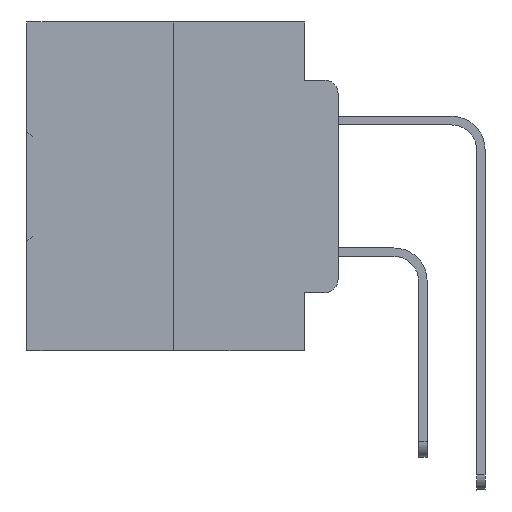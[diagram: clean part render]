
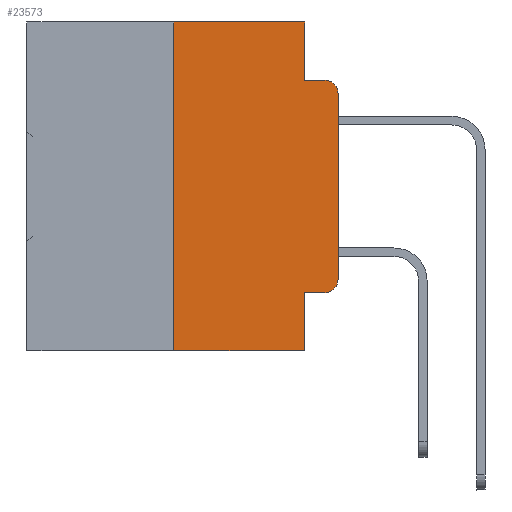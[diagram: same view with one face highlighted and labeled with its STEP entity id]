
A CAD part, left-side view. The second image highlights one B-rep face of the part: STEP entity #23573.
In plain terms, the highlighted planar face has unit normal (-1, 0, 0).
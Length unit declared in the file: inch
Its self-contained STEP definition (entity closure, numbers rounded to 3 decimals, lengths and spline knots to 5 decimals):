
#135 = CARTESIAN_POINT ( 'NONE',  ( 0., 0.25, -0.5 ) ) ;
#138 = ORIENTED_EDGE ( 'NONE', *, *, #31045, .F. ) ;
#306 = VECTOR ( 'NONE', #34280, 39.37008 ) ;
#1389 = DIRECTION ( 'NONE',  ( 0., 0., -1. ) ) ;
#1740 = LINE ( 'NONE', #16922, #306 ) ;
#2538 = LINE ( 'NONE', #29289, #10488 ) ;
#2679 = CARTESIAN_POINT ( 'NONE',  ( 0., 0.25, 0. ) ) ;
#2766 = EDGE_CURVE ( 'NONE', #17085, #12920, #2538, .T. ) ;
#3161 = ORIENTED_EDGE ( 'NONE', *, *, #13828, .T. ) ;
#3343 = VERTEX_POINT ( 'NONE', #2679 ) ;
#4258 = VERTEX_POINT ( 'NONE', #135 ) ;
#4669 = DIRECTION ( 'NONE',  ( 0., -1., 0. ) ) ;
#5214 = ORIENTED_EDGE ( 'NONE', *, *, #21017, .F. ) ;
#5657 = AXIS2_PLACEMENT_3D ( 'NONE', #33349, #15625, #1389 ) ;
#6092 = ORIENTED_EDGE ( 'NONE', *, *, #12648, .F. ) ;
#6318 = AXIS2_PLACEMENT_3D ( 'NONE', #6918, #21551, #18655 ) ;
#6918 = CARTESIAN_POINT ( 'NONE',  ( 0., 0.02, -0.1085 ) ) ;
#7199 = EDGE_CURVE ( 'NONE', #14322, #29893, #29686, .T. ) ;
#7302 = DIRECTION ( 'NONE',  ( 0., 0., 1. ) ) ;
#7470 = CARTESIAN_POINT ( 'NONE',  ( 0., 0., -0.1085 ) ) ;
#7497 = CARTESIAN_POINT ( 'NONE',  ( 0., 0.25, 0. ) ) ;
#8606 = AXIS2_PLACEMENT_3D ( 'NONE', #10008, #12335, #15586 ) ;
#10008 = CARTESIAN_POINT ( 'NONE',  ( 0., 0.473, 0. ) ) ;
#10164 = VERTEX_POINT ( 'NONE', #25922 ) ;
#10488 = VECTOR ( 'NONE', #11383, 39.37008 ) ;
#11383 = DIRECTION ( 'NONE',  ( 0., 0., -1. ) ) ;
#12335 = DIRECTION ( 'NONE',  ( 1., 0., 0. ) ) ;
#12648 = EDGE_CURVE ( 'NONE', #28767, #29893, #26604, .T. ) ;
#12920 = VERTEX_POINT ( 'NONE', #35603 ) ;
#13164 = VECTOR ( 'NONE', #18108, 39.37008 ) ;
#13828 = EDGE_CURVE ( 'NONE', #4258, #12920, #1740, .T. ) ;
#14322 = VERTEX_POINT ( 'NONE', #7470 ) ;
#15243 = EDGE_CURVE ( 'NONE', #35034, #14322, #19634, .T. ) ;
#15586 = DIRECTION ( 'NONE',  ( 0., 0., -1. ) ) ;
#15625 = DIRECTION ( 'NONE',  ( -1., 0., 0. ) ) ;
#16151 = LINE ( 'NONE', #7497, #27309 ) ;
#16922 = CARTESIAN_POINT ( 'NONE',  ( 0., 0.473, -0.5 ) ) ;
#17085 = VERTEX_POINT ( 'NONE', #23515 ) ;
#17398 = ORIENTED_EDGE ( 'NONE', *, *, #34317, .T. ) ;
#18108 = DIRECTION ( 'NONE',  ( 0., -1., 0. ) ) ;
#18655 = DIRECTION ( 'NONE',  ( 0., 0., -1. ) ) ;
#19634 = LINE ( 'NONE', #25606, #24273 ) ;
#20098 = CARTESIAN_POINT ( 'NONE',  ( 0., 0.051, 0. ) ) ;
#21001 = VERTEX_POINT ( 'NONE', #20098 ) ;
#21017 = EDGE_CURVE ( 'NONE', #3343, #21001, #29148, .T. ) ;
#21551 = DIRECTION ( 'NONE',  ( -1., 0., 0. ) ) ;
#22005 = CARTESIAN_POINT ( 'NONE',  ( 0., 0.051, -0.4115 ) ) ;
#22274 = CIRCLE ( 'NONE', #5657, 0.02 ) ;
#23018 = LINE ( 'NONE', #37488, #32980 ) ;
#23213 = EDGE_CURVE ( 'NONE', #10164, #35034, #22274, .T. ) ;
#23515 = CARTESIAN_POINT ( 'NONE',  ( 0., 0.051, -0.4115 ) ) ;
#23573 = ADVANCED_FACE ( 'NONE', ( #30215 ), #33301, .F. ) ;
#23582 = DIRECTION ( 'NONE',  ( 0., -1., 0. ) ) ;
#24273 = VECTOR ( 'NONE', #37368, 39.37008 ) ;
#24592 = CARTESIAN_POINT ( 'NONE',  ( 0., 0.02, -0.0885 ) ) ;
#25606 = CARTESIAN_POINT ( 'NONE',  ( 0., 0., 0. ) ) ;
#25759 = VECTOR ( 'NONE', #23582, 39.37008 ) ;
#25770 = ORIENTED_EDGE ( 'NONE', *, *, #2766, .F. ) ;
#25922 = CARTESIAN_POINT ( 'NONE',  ( 0., 0.02, -0.4115 ) ) ;
#26604 = LINE ( 'NONE', #35282, #13164 ) ;
#26898 = VECTOR ( 'NONE', #4669, 39.37008 ) ;
#26910 = ORIENTED_EDGE ( 'NONE', *, *, #7199, .T. ) ;
#27309 = VECTOR ( 'NONE', #7302, 39.37008 ) ;
#27377 = EDGE_LOOP ( 'NONE', ( #36675, #26910, #6092, #138, #5214, #34987, #3161, #25770, #17398, #30146 ) ) ;
#27775 = LINE ( 'NONE', #22005, #26898 ) ;
#28227 = DIRECTION ( 'NONE',  ( 0., 0., -1. ) ) ;
#28767 = VERTEX_POINT ( 'NONE', #30829 ) ;
#28963 = CARTESIAN_POINT ( 'NONE',  ( 0., 0.473, 0. ) ) ;
#29109 = EDGE_CURVE ( 'NONE', #4258, #3343, #16151, .T. ) ;
#29148 = LINE ( 'NONE', #28963, #25759 ) ;
#29289 = CARTESIAN_POINT ( 'NONE',  ( 0., 0.051, 0. ) ) ;
#29440 = CARTESIAN_POINT ( 'NONE',  ( 0., 0., -0.3915 ) ) ;
#29686 = CIRCLE ( 'NONE', #6318, 0.02 ) ;
#29893 = VERTEX_POINT ( 'NONE', #24592 ) ;
#30146 = ORIENTED_EDGE ( 'NONE', *, *, #23213, .T. ) ;
#30215 = FACE_OUTER_BOUND ( 'NONE', #27377, .T. ) ;
#30829 = CARTESIAN_POINT ( 'NONE',  ( 0., 0.051, -0.0885 ) ) ;
#31045 = EDGE_CURVE ( 'NONE', #21001, #28767, #23018, .T. ) ;
#32980 = VECTOR ( 'NONE', #28227, 39.37008 ) ;
#33301 = PLANE ( 'NONE',  #8606 ) ;
#33349 = CARTESIAN_POINT ( 'NONE',  ( 0., 0.02, -0.3915 ) ) ;
#34280 = DIRECTION ( 'NONE',  ( 0., -1., 0. ) ) ;
#34317 = EDGE_CURVE ( 'NONE', #17085, #10164, #27775, .T. ) ;
#34987 = ORIENTED_EDGE ( 'NONE', *, *, #29109, .F. ) ;
#35034 = VERTEX_POINT ( 'NONE', #29440 ) ;
#35282 = CARTESIAN_POINT ( 'NONE',  ( 0., 0.051, -0.0885 ) ) ;
#35603 = CARTESIAN_POINT ( 'NONE',  ( 0., 0.051, -0.5 ) ) ;
#36675 = ORIENTED_EDGE ( 'NONE', *, *, #15243, .T. ) ;
#37368 = DIRECTION ( 'NONE',  ( 0., 0., 1. ) ) ;
#37488 = CARTESIAN_POINT ( 'NONE',  ( 0., 0.051, 0. ) ) ;
